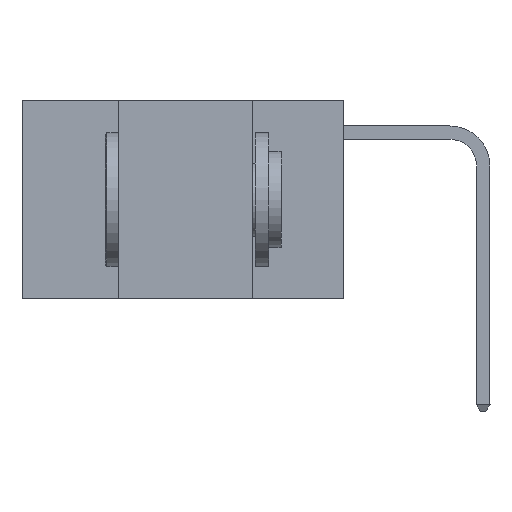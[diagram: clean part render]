
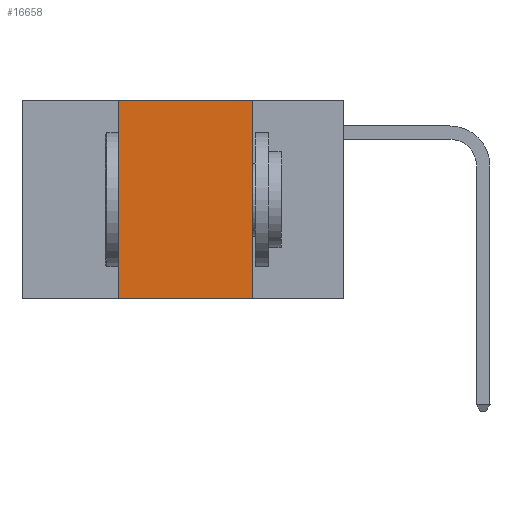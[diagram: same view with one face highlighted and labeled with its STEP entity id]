
A CAD part, left-side view. The second image highlights one B-rep face of the part: STEP entity #16658.
In plain terms, the highlighted planar face has unit normal (-1, 0, 0).
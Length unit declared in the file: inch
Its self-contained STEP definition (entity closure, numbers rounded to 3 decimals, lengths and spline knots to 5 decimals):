
#3159 = VECTOR ( 'NONE', #5679, 39.37008 ) ;
#4220 = EDGE_CURVE ( 'NONE', #12622, #28708, #16758, .T. ) ;
#5679 = DIRECTION ( 'NONE',  ( 0., -1., 0. ) ) ;
#5828 = DIRECTION ( 'NONE',  ( 0., 0., -1. ) ) ;
#7124 = CARTESIAN_POINT ( 'NONE',  ( 0., 0.17, -0.37 ) ) ;
#9053 = DIRECTION ( 'NONE',  ( 0., 0., -1. ) ) ;
#11037 = VERTEX_POINT ( 'NONE', #7124 ) ;
#12019 = CARTESIAN_POINT ( 'NONE',  ( 0., 0.42, 0. ) ) ;
#12341 = CARTESIAN_POINT ( 'NONE',  ( 0., 0.17, 0. ) ) ;
#12622 = VERTEX_POINT ( 'NONE', #27467 ) ;
#13059 = EDGE_CURVE ( 'NONE', #12622, #11037, #13833, .T. ) ;
#13833 = LINE ( 'NONE', #19962, #3159 ) ;
#14597 = DIRECTION ( 'NONE',  ( 0., 0., 1. ) ) ;
#15161 = LINE ( 'NONE', #25080, #25749 ) ;
#15663 = ORIENTED_EDGE ( 'NONE', *, *, #4220, .F. ) ;
#15706 = AXIS2_PLACEMENT_3D ( 'NONE', #20694, #16037, #9053 ) ;
#15939 = EDGE_LOOP ( 'NONE', ( #16773, #19814, #15663, #25817 ) ) ;
#16037 = DIRECTION ( 'NONE',  ( 1., 0., 0. ) ) ;
#16658 = ADVANCED_FACE ( 'NONE', ( #25681 ), #20845, .F. ) ;
#16758 = LINE ( 'NONE', #19252, #24902 ) ;
#16773 = ORIENTED_EDGE ( 'NONE', *, *, #28407, .F. ) ;
#17661 = VERTEX_POINT ( 'NONE', #12341 ) ;
#19252 = CARTESIAN_POINT ( 'NONE',  ( 0., 0.42, 0. ) ) ;
#19814 = ORIENTED_EDGE ( 'NONE', *, *, #24263, .F. ) ;
#19962 = CARTESIAN_POINT ( 'NONE',  ( 0., 0.6, -0.37 ) ) ;
#20460 = LINE ( 'NONE', #20607, #22851 ) ;
#20607 = CARTESIAN_POINT ( 'NONE',  ( 0., 0.6, 0. ) ) ;
#20694 = CARTESIAN_POINT ( 'NONE',  ( 0., 0.6, 0. ) ) ;
#20845 = PLANE ( 'NONE',  #15706 ) ;
#22851 = VECTOR ( 'NONE', #25287, 39.37008 ) ;
#24263 = EDGE_CURVE ( 'NONE', #28708, #17661, #20460, .T. ) ;
#24902 = VECTOR ( 'NONE', #14597, 39.37008 ) ;
#25080 = CARTESIAN_POINT ( 'NONE',  ( 0., 0.17, 0. ) ) ;
#25287 = DIRECTION ( 'NONE',  ( 0., -1., 0. ) ) ;
#25681 = FACE_OUTER_BOUND ( 'NONE', #15939, .T. ) ;
#25749 = VECTOR ( 'NONE', #5828, 39.37008 ) ;
#25817 = ORIENTED_EDGE ( 'NONE', *, *, #13059, .T. ) ;
#27467 = CARTESIAN_POINT ( 'NONE',  ( 0., 0.42, -0.37 ) ) ;
#28407 = EDGE_CURVE ( 'NONE', #17661, #11037, #15161, .T. ) ;
#28708 = VERTEX_POINT ( 'NONE', #12019 ) ;
